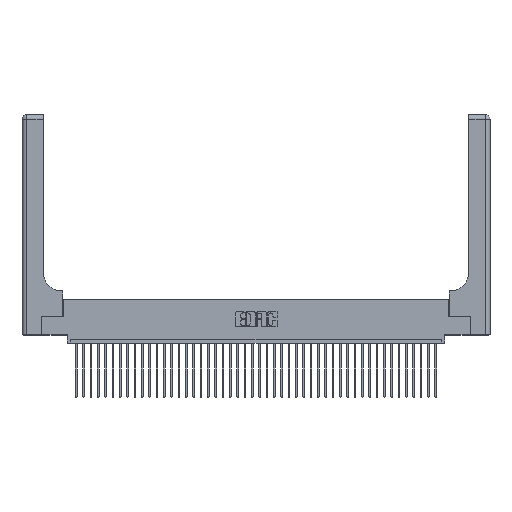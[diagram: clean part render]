
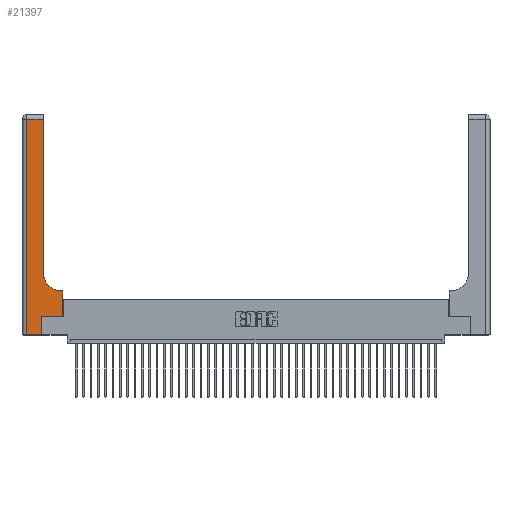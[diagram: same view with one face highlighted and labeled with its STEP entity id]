
A CAD part, top view. The second image highlights one B-rep face of the part: STEP entity #21397.
In plain terms, the highlighted planar face has unit normal (0, 0, 1).
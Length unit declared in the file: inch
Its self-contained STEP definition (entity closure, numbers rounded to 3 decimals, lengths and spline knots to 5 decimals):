
#1514 = EDGE_LOOP ( 'NONE', ( #13066, #23138, #31966, #28168, #8247, #9077, #3360, #7620, #14393 ) ) ;
#2333 = LINE ( 'NONE', #5366, #8397 ) ;
#2586 = VECTOR ( 'NONE', #34644, 39.37008 ) ;
#3360 = ORIENTED_EDGE ( 'NONE', *, *, #12658, .T. ) ;
#4478 = DIRECTION ( 'NONE',  ( 1., 0., 0. ) ) ;
#5366 = CARTESIAN_POINT ( 'NONE',  ( 0.2915, 0.6, 0.37 ) ) ;
#5510 = DIRECTION ( 'NONE',  ( -1., 0., 0. ) ) ;
#6646 = EDGE_CURVE ( 'NONE', #32862, #21507, #40473, .T. ) ;
#7616 = CARTESIAN_POINT ( 'NONE',  ( 0.269, 0.25, 0.37 ) ) ;
#7620 = ORIENTED_EDGE ( 'NONE', *, *, #9396, .T. ) ;
#8060 = EDGE_CURVE ( 'NONE', #26806, #21815, #35323, .T. ) ;
#8247 = ORIENTED_EDGE ( 'NONE', *, *, #15862, .T. ) ;
#8397 = VECTOR ( 'NONE', #5510, 39.37008 ) ;
#9077 = ORIENTED_EDGE ( 'NONE', *, *, #41016, .T. ) ;
#9338 = DIRECTION ( 'NONE',  ( 1., 0., 0. ) ) ;
#9396 = EDGE_CURVE ( 'NONE', #31890, #18648, #2333, .T. ) ;
#10469 = CARTESIAN_POINT ( 'NONE',  ( 0.2915, 0.85, 0.37 ) ) ;
#10977 = CARTESIAN_POINT ( 'NONE',  ( 0.5585, 0.25, 0.37 ) ) ;
#11023 = VECTOR ( 'NONE', #21388, 39.37008 ) ;
#11829 = CARTESIAN_POINT ( 'NONE',  ( 0.2915, 3., 0.37 ) ) ;
#12658 = EDGE_CURVE ( 'NONE', #15942, #31890, #26269, .T. ) ;
#13066 = ORIENTED_EDGE ( 'NONE', *, *, #8060, .T. ) ;
#14393 = ORIENTED_EDGE ( 'NONE', *, *, #39619, .T. ) ;
#14574 = CARTESIAN_POINT ( 'NONE',  ( 0.5585, 0.6, 0.37 ) ) ;
#15642 = DIRECTION ( 'NONE',  ( -1., 0., 0. ) ) ;
#15714 = DIRECTION ( 'NONE',  ( 0., 0., -1. ) ) ;
#15862 = EDGE_CURVE ( 'NONE', #21507, #41749, #25177, .T. ) ;
#15942 = VERTEX_POINT ( 'NONE', #10977 ) ;
#16230 = DIRECTION ( 'NONE',  ( -1., 0., 0. ) ) ;
#16387 = VERTEX_POINT ( 'NONE', #28309 ) ;
#17146 = LINE ( 'NONE', #35584, #34370 ) ;
#18248 = LINE ( 'NONE', #7616, #31840 ) ;
#18648 = VERTEX_POINT ( 'NONE', #27032 ) ;
#18767 = AXIS2_PLACEMENT_3D ( 'NONE', #26675, #36480, #15642 ) ;
#20156 = VECTOR ( 'NONE', #30305, 39.37008 ) ;
#21041 = CARTESIAN_POINT ( 'NONE',  ( 0.2915, 2.94, 0.37 ) ) ;
#21388 = DIRECTION ( 'NONE',  ( 0., -1., 0. ) ) ;
#21395 = DIRECTION ( 'NONE',  ( 0., 1., 0. ) ) ;
#21397 = ADVANCED_FACE ( 'NONE', ( #38677 ), #40809, .F. ) ;
#21507 = VERTEX_POINT ( 'NONE', #21843 ) ;
#21815 = VERTEX_POINT ( 'NONE', #21041 ) ;
#21843 = CARTESIAN_POINT ( 'NONE',  ( 0.269, 0., 0.37 ) ) ;
#22176 = VECTOR ( 'NONE', #21395, 39.37008 ) ;
#22558 = CARTESIAN_POINT ( 'NONE',  ( 0.5415, 0.85, 0.37 ) ) ;
#23138 = ORIENTED_EDGE ( 'NONE', *, *, #41302, .T. ) ;
#23590 = LINE ( 'NONE', #28143, #11023 ) ;
#25177 = LINE ( 'NONE', #33278, #40921 ) ;
#26269 = LINE ( 'NONE', #32274, #2586 ) ;
#26675 = CARTESIAN_POINT ( 'NONE',  ( 0., 3., 0.37 ) ) ;
#26806 = VERTEX_POINT ( 'NONE', #10469 ) ;
#26869 = CIRCLE ( 'NONE', #41389, 0.25 ) ;
#27032 = CARTESIAN_POINT ( 'NONE',  ( 0.5415, 0.6, 0.37 ) ) ;
#28143 = CARTESIAN_POINT ( 'NONE',  ( 0.06, 3., 0.37 ) ) ;
#28168 = ORIENTED_EDGE ( 'NONE', *, *, #6646, .T. ) ;
#28309 = CARTESIAN_POINT ( 'NONE',  ( 0.06, 2.94, 0.37 ) ) ;
#29543 = DIRECTION ( 'NONE',  ( 0., 1., 0. ) ) ;
#30305 = DIRECTION ( 'NONE',  ( 1., 0., 0. ) ) ;
#30535 = EDGE_CURVE ( 'NONE', #16387, #32862, #23590, .T. ) ;
#31840 = VECTOR ( 'NONE', #4478, 39.37008 ) ;
#31890 = VERTEX_POINT ( 'NONE', #14574 ) ;
#31966 = ORIENTED_EDGE ( 'NONE', *, *, #30535, .T. ) ;
#32274 = CARTESIAN_POINT ( 'NONE',  ( 0.5585, 0.25, 0.37 ) ) ;
#32862 = VERTEX_POINT ( 'NONE', #36625 ) ;
#33267 = CARTESIAN_POINT ( 'NONE',  ( 0., 0., 0.37 ) ) ;
#33278 = CARTESIAN_POINT ( 'NONE',  ( 0.269, 0., 0.37 ) ) ;
#34370 = VECTOR ( 'NONE', #16230, 39.37008 ) ;
#34644 = DIRECTION ( 'NONE',  ( 0., 1., 0. ) ) ;
#35323 = LINE ( 'NONE', #11829, #22176 ) ;
#35584 = CARTESIAN_POINT ( 'NONE',  ( 0., 2.94, 0.37 ) ) ;
#36480 = DIRECTION ( 'NONE',  ( 0., 0., -1. ) ) ;
#36625 = CARTESIAN_POINT ( 'NONE',  ( 0.06, 0., 0.37 ) ) ;
#38677 = FACE_OUTER_BOUND ( 'NONE', #1514, .T. ) ;
#39144 = CARTESIAN_POINT ( 'NONE',  ( 0.269, 0.25, 0.37 ) ) ;
#39619 = EDGE_CURVE ( 'NONE', #18648, #26806, #26869, .T. ) ;
#40473 = LINE ( 'NONE', #33267, #20156 ) ;
#40809 = PLANE ( 'NONE',  #18767 ) ;
#40921 = VECTOR ( 'NONE', #29543, 39.37008 ) ;
#41016 = EDGE_CURVE ( 'NONE', #41749, #15942, #18248, .T. ) ;
#41302 = EDGE_CURVE ( 'NONE', #21815, #16387, #17146, .T. ) ;
#41389 = AXIS2_PLACEMENT_3D ( 'NONE', #22558, #15714, #9338 ) ;
#41749 = VERTEX_POINT ( 'NONE', #39144 ) ;
